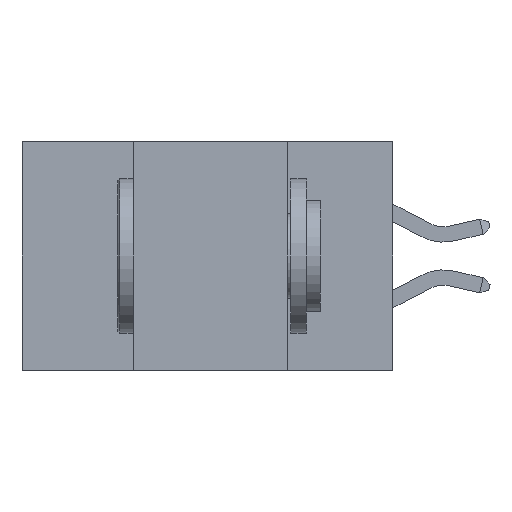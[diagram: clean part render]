
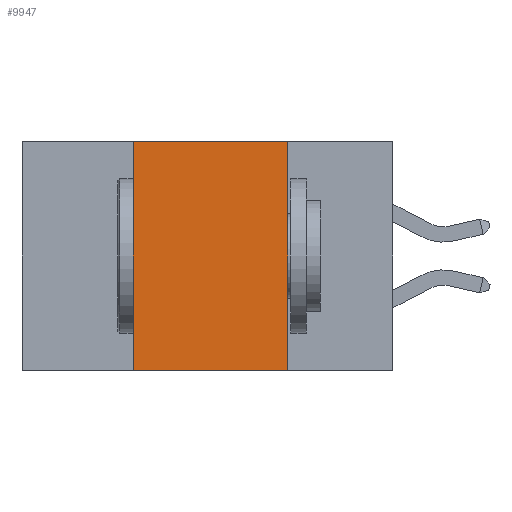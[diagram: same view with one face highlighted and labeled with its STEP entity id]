
A CAD part, left-side view. The second image highlights one B-rep face of the part: STEP entity #9947.
In plain terms, the highlighted planar face has unit normal (-1, 0, 0).
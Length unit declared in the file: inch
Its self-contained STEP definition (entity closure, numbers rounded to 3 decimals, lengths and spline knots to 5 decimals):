
#370 = CARTESIAN_POINT ( 'NONE',  ( 0., 0.42, 0. ) ) ;
#499 = CARTESIAN_POINT ( 'NONE',  ( 0., 0.17, -0.37 ) ) ;
#776 = DIRECTION ( 'NONE',  ( 1., 0., 0. ) ) ;
#890 = AXIS2_PLACEMENT_3D ( 'NONE', #5654, #776, #10379 ) ;
#1005 = ORIENTED_EDGE ( 'NONE', *, *, #4897, .T. ) ;
#2444 = LINE ( 'NONE', #14564, #11241 ) ;
#3023 = PLANE ( 'NONE',  #890 ) ;
#3597 = EDGE_LOOP ( 'NONE', ( #11490, #6775, #11795, #1005 ) ) ;
#4136 = VECTOR ( 'NONE', #11467, 39.37008 ) ;
#4897 = EDGE_CURVE ( 'NONE', #12886, #10461, #2444, .T. ) ;
#5586 = FACE_OUTER_BOUND ( 'NONE', #3597, .T. ) ;
#5654 = CARTESIAN_POINT ( 'NONE',  ( 0., 0.6, 0. ) ) ;
#6775 = ORIENTED_EDGE ( 'NONE', *, *, #9237, .F. ) ;
#6960 = VERTEX_POINT ( 'NONE', #8422 ) ;
#7940 = CARTESIAN_POINT ( 'NONE',  ( 0., 0.6, 0. ) ) ;
#8422 = CARTESIAN_POINT ( 'NONE',  ( 0., 0.17, 0. ) ) ;
#8548 = LINE ( 'NONE', #12199, #12372 ) ;
#9032 = CARTESIAN_POINT ( 'NONE',  ( 0., 0.42, 0. ) ) ;
#9237 = EDGE_CURVE ( 'NONE', #10982, #6960, #12889, .T. ) ;
#9947 = ADVANCED_FACE ( 'NONE', ( #5586 ), #3023, .F. ) ;
#10361 = CARTESIAN_POINT ( 'NONE',  ( 0., 0.42, -0.37 ) ) ;
#10379 = DIRECTION ( 'NONE',  ( 0., 0., -1. ) ) ;
#10396 = DIRECTION ( 'NONE',  ( 0., -1., 0. ) ) ;
#10461 = VERTEX_POINT ( 'NONE', #499 ) ;
#10982 = VERTEX_POINT ( 'NONE', #9032 ) ;
#11241 = VECTOR ( 'NONE', #13358, 39.37008 ) ;
#11467 = DIRECTION ( 'NONE',  ( 0., 0., 1. ) ) ;
#11490 = ORIENTED_EDGE ( 'NONE', *, *, #14521, .F. ) ;
#11795 = ORIENTED_EDGE ( 'NONE', *, *, #13471, .F. ) ;
#12199 = CARTESIAN_POINT ( 'NONE',  ( 0., 0.17, 0. ) ) ;
#12372 = VECTOR ( 'NONE', #15734, 39.37008 ) ;
#12886 = VERTEX_POINT ( 'NONE', #10361 ) ;
#12889 = LINE ( 'NONE', #7940, #14964 ) ;
#13358 = DIRECTION ( 'NONE',  ( 0., -1., 0. ) ) ;
#13471 = EDGE_CURVE ( 'NONE', #12886, #10982, #13910, .T. ) ;
#13910 = LINE ( 'NONE', #370, #4136 ) ;
#14521 = EDGE_CURVE ( 'NONE', #6960, #10461, #8548, .T. ) ;
#14564 = CARTESIAN_POINT ( 'NONE',  ( 0., 0.6, -0.37 ) ) ;
#14964 = VECTOR ( 'NONE', #10396, 39.37008 ) ;
#15734 = DIRECTION ( 'NONE',  ( 0., 0., -1. ) ) ;
